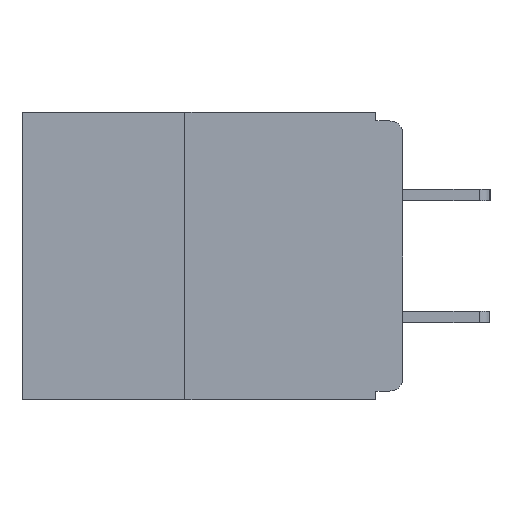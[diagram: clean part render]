
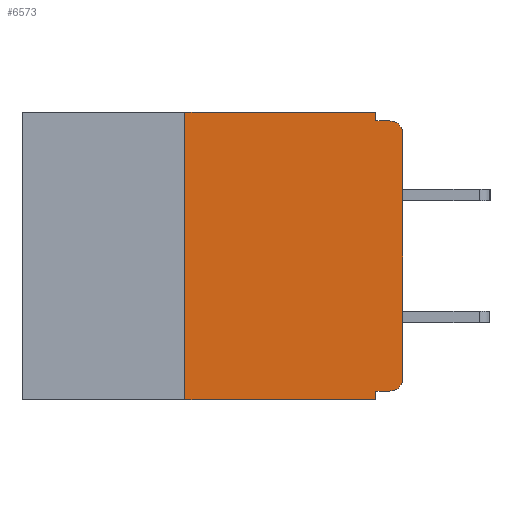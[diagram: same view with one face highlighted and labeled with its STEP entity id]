
A CAD part, left-side view. The second image highlights one B-rep face of the part: STEP entity #6573.
In plain terms, the highlighted planar face has unit normal (-1, 0, 0).
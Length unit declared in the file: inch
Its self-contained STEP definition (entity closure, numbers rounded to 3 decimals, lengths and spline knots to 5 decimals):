
#22 = LINE ( 'NONE', #12643, #8978 ) ;
#137 = CARTESIAN_POINT ( 'NONE',  ( 0., 0., 0. ) ) ;
#195 = VERTEX_POINT ( 'NONE', #2526 ) ;
#198 = VERTEX_POINT ( 'NONE', #8406 ) ;
#208 = VERTEX_POINT ( 'NONE', #9821 ) ;
#248 = CARTESIAN_POINT ( 'NONE',  ( 0., 0.437, 0. ) ) ;
#252 = CARTESIAN_POINT ( 'NONE',  ( 0., 0., -0.32 ) ) ;
#362 = CARTESIAN_POINT ( 'NONE',  ( 0., 0.031, 0. ) ) ;
#604 = VERTEX_POINT ( 'NONE', #7199 ) ;
#987 = DIRECTION ( 'NONE',  ( 0., 0., -1. ) ) ;
#1095 = EDGE_CURVE ( 'NONE', #604, #8852, #11356, .T. ) ;
#1520 = DIRECTION ( 'NONE',  ( 0., 0., -1. ) ) ;
#1603 = ORIENTED_EDGE ( 'NONE', *, *, #12379, .T. ) ;
#1633 = VECTOR ( 'NONE', #13467, 39.37008 ) ;
#1773 = ORIENTED_EDGE ( 'NONE', *, *, #8200, .T. ) ;
#2025 = DIRECTION ( 'NONE',  ( 0., 0., 1. ) ) ;
#2260 = ORIENTED_EDGE ( 'NONE', *, *, #9858, .F. ) ;
#2526 = CARTESIAN_POINT ( 'NONE',  ( 0., 0., -0.305 ) ) ;
#2687 = LINE ( 'NONE', #5331, #3404 ) ;
#3119 = LINE ( 'NONE', #4028, #8673 ) ;
#3273 = ORIENTED_EDGE ( 'NONE', *, *, #10762, .T. ) ;
#3404 = VECTOR ( 'NONE', #4173, 39.37008 ) ;
#3695 = ORIENTED_EDGE ( 'NONE', *, *, #12054, .T. ) ;
#4028 = CARTESIAN_POINT ( 'NONE',  ( 0., 0.031, -0.33 ) ) ;
#4054 = DIRECTION ( 'NONE',  ( 0., 0., -1. ) ) ;
#4173 = DIRECTION ( 'NONE',  ( 0., -1., 0. ) ) ;
#4409 = CIRCLE ( 'NONE', #6468, 0.015 ) ;
#4439 = VECTOR ( 'NONE', #1520, 39.37008 ) ;
#4720 = LINE ( 'NONE', #137, #1633 ) ;
#5203 = EDGE_CURVE ( 'NONE', #8852, #13713, #3119, .T. ) ;
#5331 = CARTESIAN_POINT ( 'NONE',  ( 0., 0.437, -0.33 ) ) ;
#5575 = EDGE_CURVE ( 'NONE', #208, #13655, #22, .T. ) ;
#5634 = CARTESIAN_POINT ( 'NONE',  ( 0., 0.437, 0. ) ) ;
#5773 = ORIENTED_EDGE ( 'NONE', *, *, #1095, .F. ) ;
#6468 = AXIS2_PLACEMENT_3D ( 'NONE', #6591, #14155, #7666 ) ;
#6573 = ADVANCED_FACE ( 'NONE', ( #9281 ), #6694, .F. ) ;
#6591 = CARTESIAN_POINT ( 'NONE',  ( 0., 0.015, -0.305 ) ) ;
#6694 = PLANE ( 'NONE',  #11933 ) ;
#6735 = DIRECTION ( 'NONE',  ( 0., 0., -1. ) ) ;
#6756 = EDGE_CURVE ( 'NONE', #12711, #198, #6878, .T. ) ;
#6878 = LINE ( 'NONE', #248, #12351 ) ;
#7199 = CARTESIAN_POINT ( 'NONE',  ( 0., 0.015, -0.32 ) ) ;
#7203 = DIRECTION ( 'NONE',  ( 0., -1., 0. ) ) ;
#7416 = ORIENTED_EDGE ( 'NONE', *, *, #6756, .F. ) ;
#7643 = CARTESIAN_POINT ( 'NONE',  ( 0., 0.25, -0.33 ) ) ;
#7666 = DIRECTION ( 'NONE',  ( 0., 0., -1. ) ) ;
#7718 = DIRECTION ( 'NONE',  ( -1., 0., 0. ) ) ;
#8143 = CIRCLE ( 'NONE', #12424, 0.015 ) ;
#8200 = EDGE_CURVE ( 'NONE', #10080, #13713, #2687, .T. ) ;
#8201 = DIRECTION ( 'NONE',  ( 0., 1., 0. ) ) ;
#8290 = EDGE_CURVE ( 'NONE', #10080, #12711, #12995, .T. ) ;
#8380 = ORIENTED_EDGE ( 'NONE', *, *, #5575, .F. ) ;
#8406 = CARTESIAN_POINT ( 'NONE',  ( 0., 0.031, 0. ) ) ;
#8443 = VECTOR ( 'NONE', #8201, 39.37008 ) ;
#8673 = VECTOR ( 'NONE', #4054, 39.37008 ) ;
#8852 = VERTEX_POINT ( 'NONE', #12044 ) ;
#8978 = VECTOR ( 'NONE', #7203, 39.37008 ) ;
#9281 = FACE_OUTER_BOUND ( 'NONE', #11553, .T. ) ;
#9286 = ORIENTED_EDGE ( 'NONE', *, *, #5203, .F. ) ;
#9821 = CARTESIAN_POINT ( 'NONE',  ( 0., 0.031, -0.01 ) ) ;
#9858 = EDGE_CURVE ( 'NONE', #198, #208, #10267, .T. ) ;
#9908 = ORIENTED_EDGE ( 'NONE', *, *, #8290, .F. ) ;
#10080 = VERTEX_POINT ( 'NONE', #10834 ) ;
#10143 = VECTOR ( 'NONE', #2025, 39.37008 ) ;
#10267 = LINE ( 'NONE', #362, #4439 ) ;
#10762 = EDGE_CURVE ( 'NONE', #604, #195, #4409, .T. ) ;
#10834 = CARTESIAN_POINT ( 'NONE',  ( 0., 0.25, -0.33 ) ) ;
#11218 = VERTEX_POINT ( 'NONE', #12729 ) ;
#11356 = LINE ( 'NONE', #252, #8443 ) ;
#11553 = EDGE_LOOP ( 'NONE', ( #3695, #1603, #8380, #2260, #7416, #9908, #1773, #9286, #5773, #3273 ) ) ;
#11612 = CARTESIAN_POINT ( 'NONE',  ( 0., 0.25, 0. ) ) ;
#11933 = AXIS2_PLACEMENT_3D ( 'NONE', #5634, #13244, #6735 ) ;
#12044 = CARTESIAN_POINT ( 'NONE',  ( 0., 0.031, -0.32 ) ) ;
#12054 = EDGE_CURVE ( 'NONE', #195, #11218, #4720, .T. ) ;
#12138 = CARTESIAN_POINT ( 'NONE',  ( 0., 0.015, -0.01 ) ) ;
#12351 = VECTOR ( 'NONE', #13522, 39.37008 ) ;
#12379 = EDGE_CURVE ( 'NONE', #11218, #13655, #8143, .T. ) ;
#12424 = AXIS2_PLACEMENT_3D ( 'NONE', #14197, #7718, #987 ) ;
#12643 = CARTESIAN_POINT ( 'NONE',  ( 0., 0., -0.01 ) ) ;
#12711 = VERTEX_POINT ( 'NONE', #11612 ) ;
#12729 = CARTESIAN_POINT ( 'NONE',  ( 0., 0., -0.025 ) ) ;
#12995 = LINE ( 'NONE', #7643, #10143 ) ;
#13244 = DIRECTION ( 'NONE',  ( 1., 0., 0. ) ) ;
#13282 = CARTESIAN_POINT ( 'NONE',  ( 0., 0.031, -0.33 ) ) ;
#13467 = DIRECTION ( 'NONE',  ( 0., 0., 1. ) ) ;
#13522 = DIRECTION ( 'NONE',  ( 0., -1., 0. ) ) ;
#13655 = VERTEX_POINT ( 'NONE', #12138 ) ;
#13713 = VERTEX_POINT ( 'NONE', #13282 ) ;
#14155 = DIRECTION ( 'NONE',  ( -1., 0., 0. ) ) ;
#14197 = CARTESIAN_POINT ( 'NONE',  ( 0., 0.015, -0.025 ) ) ;
